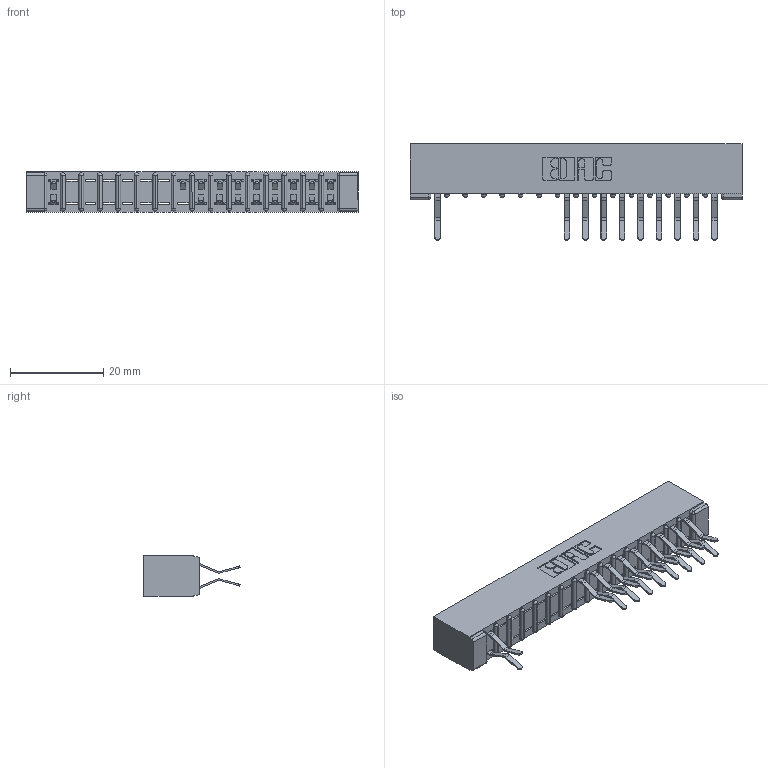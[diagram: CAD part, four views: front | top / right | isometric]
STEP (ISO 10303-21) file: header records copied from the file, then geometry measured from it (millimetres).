
FILE_DESCRIPTION (( 'STEP AP203' ), '1' );
FILE_NAME ('307-032-560-201.STEP', '2018-08-04T22:59:34', ( '' ), ( '' ), 'SwSTEP 2.0', 'SolidWorks 2016', '' );
FILE_SCHEMA (( 'CONFIG_CONTROL_DESIGN' ));
Length unit declared in the file: inch
Products named in the file (3): 307 Part_No Mounting Lugs; 307-290-001_560; 307-032-560-201
Assembly tree (20 placements, depth 2):
  307-032-560-201
    307 Part_No Mounting Lugs
    307-290-001_560  x19
Bounding box: 71.27 x 20.73 x 8.71 mm (x, y, z)
Volume: 4751.1 mm3; surface area: 7699.3 mm2
Topology: 20 solids, 20 shells, 1207 faces, 3413 edges, 2202 vertices
Faces by surface type: plane 771, cylinder 402, sphere 34
Entity records: 16844 total; most frequent: CARTESIAN_POINT 2815, ORIENTED_EDGE 2798, DIRECTION 2755, EDGE_CURVE 1399, LINE 1063, VECTOR 1063, VERTEX_POINT 906, AXIS2_PLACEMENT_3D 846
